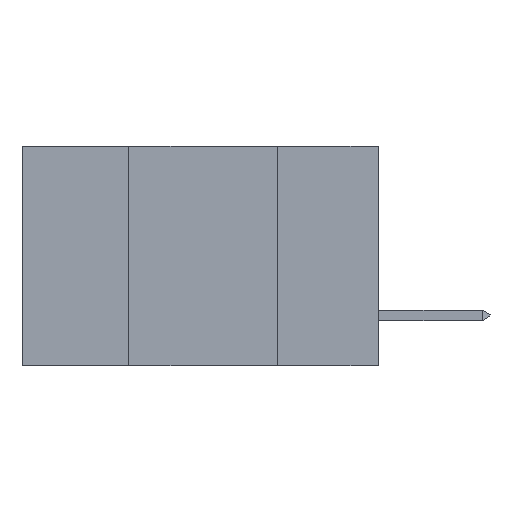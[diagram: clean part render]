
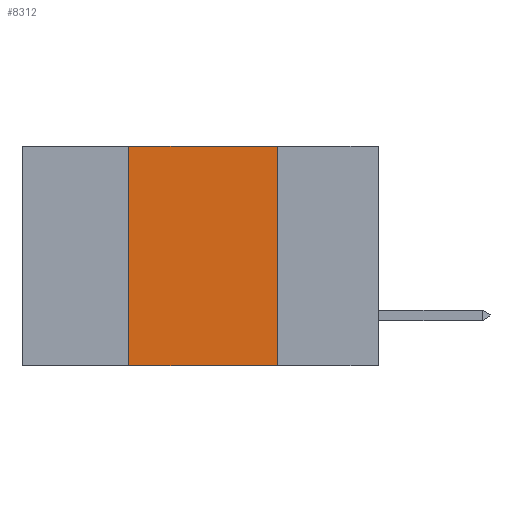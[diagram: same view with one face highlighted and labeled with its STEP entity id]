
A CAD part, left-side view. The second image highlights one B-rep face of the part: STEP entity #8312.
In plain terms, the highlighted planar face has unit normal (-1, 0, 0).
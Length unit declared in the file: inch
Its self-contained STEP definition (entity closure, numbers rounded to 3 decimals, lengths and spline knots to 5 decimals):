
#180 = VERTEX_POINT ( 'NONE', #12128 ) ;
#717 = CARTESIAN_POINT ( 'NONE',  ( 0., 0.42, 0. ) ) ;
#766 = DIRECTION ( 'NONE',  ( 0., 0., 1. ) ) ;
#969 = EDGE_CURVE ( 'NONE', #14750, #180, #7663, .T. ) ;
#2038 = VECTOR ( 'NONE', #766, 39.37008 ) ;
#2344 = CARTESIAN_POINT ( 'NONE',  ( 0., 0.6, 0. ) ) ;
#2811 = VECTOR ( 'NONE', #3869, 39.37008 ) ;
#2827 = FACE_OUTER_BOUND ( 'NONE', #6862, .T. ) ;
#3791 = LINE ( 'NONE', #2344, #2811 ) ;
#3869 = DIRECTION ( 'NONE',  ( 0., -1., 0. ) ) ;
#4343 = VECTOR ( 'NONE', #13279, 39.37008 ) ;
#4740 = CARTESIAN_POINT ( 'NONE',  ( 0., 0.17, -0.37 ) ) ;
#4753 = EDGE_CURVE ( 'NONE', #7437, #8834, #3791, .T. ) ;
#4952 = DIRECTION ( 'NONE',  ( 1., 0., 0. ) ) ;
#5103 = PLANE ( 'NONE',  #10579 ) ;
#5770 = LINE ( 'NONE', #9382, #2038 ) ;
#6224 = DIRECTION ( 'NONE',  ( 0., 0., -1. ) ) ;
#6862 = EDGE_LOOP ( 'NONE', ( #13161, #14634, #12725, #8545 ) ) ;
#7437 = VERTEX_POINT ( 'NONE', #717 ) ;
#7590 = DIRECTION ( 'NONE',  ( 0., -1., 0. ) ) ;
#7663 = LINE ( 'NONE', #15166, #10204 ) ;
#8312 = ADVANCED_FACE ( 'NONE', ( #2827 ), #5103, .F. ) ;
#8545 = ORIENTED_EDGE ( 'NONE', *, *, #969, .T. ) ;
#8834 = VERTEX_POINT ( 'NONE', #9906 ) ;
#9382 = CARTESIAN_POINT ( 'NONE',  ( 0., 0.42, -0.37 ) ) ;
#9492 = EDGE_CURVE ( 'NONE', #8834, #180, #12153, .T. ) ;
#9906 = CARTESIAN_POINT ( 'NONE',  ( 0., 0.17, 0. ) ) ;
#10204 = VECTOR ( 'NONE', #7590, 39.37008 ) ;
#10579 = AXIS2_PLACEMENT_3D ( 'NONE', #14967, #4952, #6224 ) ;
#10931 = EDGE_CURVE ( 'NONE', #14750, #7437, #5770, .T. ) ;
#12128 = CARTESIAN_POINT ( 'NONE',  ( 0., 0.17, -0.37 ) ) ;
#12153 = LINE ( 'NONE', #4740, #4343 ) ;
#12725 = ORIENTED_EDGE ( 'NONE', *, *, #10931, .F. ) ;
#13161 = ORIENTED_EDGE ( 'NONE', *, *, #9492, .F. ) ;
#13279 = DIRECTION ( 'NONE',  ( 0., 0., -1. ) ) ;
#13924 = CARTESIAN_POINT ( 'NONE',  ( 0., 0.42, -0.37 ) ) ;
#14634 = ORIENTED_EDGE ( 'NONE', *, *, #4753, .F. ) ;
#14750 = VERTEX_POINT ( 'NONE', #13924 ) ;
#14967 = CARTESIAN_POINT ( 'NONE',  ( 0., 0.6, 0. ) ) ;
#15166 = CARTESIAN_POINT ( 'NONE',  ( 0., 0.6, -0.37 ) ) ;
